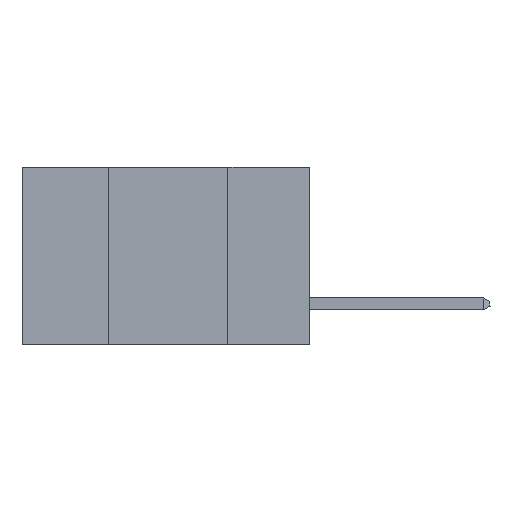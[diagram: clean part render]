
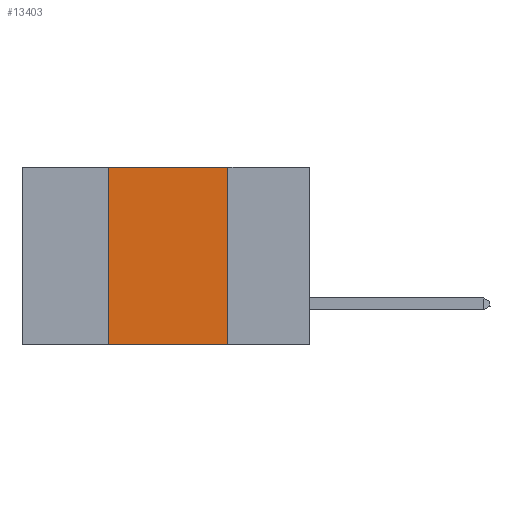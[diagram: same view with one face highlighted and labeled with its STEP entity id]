
A CAD part, left-side view. The second image highlights one B-rep face of the part: STEP entity #13403.
In plain terms, the highlighted planar face has unit normal (-1, 0, 0).
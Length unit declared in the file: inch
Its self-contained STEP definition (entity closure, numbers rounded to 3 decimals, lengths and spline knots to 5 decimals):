
#930 = EDGE_CURVE ( 'NONE', #6427, #4068, #12873, .T. ) ;
#1268 = PLANE ( 'NONE',  #1654 ) ;
#1447 = DIRECTION ( 'NONE',  ( 0., 0., 1. ) ) ;
#1532 = CARTESIAN_POINT ( 'NONE',  ( 0., 0.42, 0. ) ) ;
#1654 = AXIS2_PLACEMENT_3D ( 'NONE', #4672, #16236, #6353 ) ;
#1866 = VECTOR ( 'NONE', #7401, 39.37008 ) ;
#2319 = CARTESIAN_POINT ( 'NONE',  ( 0., 0.6, 0. ) ) ;
#2408 = VERTEX_POINT ( 'NONE', #3628 ) ;
#2888 = VECTOR ( 'NONE', #15677, 39.37008 ) ;
#2890 = EDGE_LOOP ( 'NONE', ( #3786, #19880, #3697, #14132 ) ) ;
#3628 = CARTESIAN_POINT ( 'NONE',  ( 0., 0.17, 0. ) ) ;
#3697 = ORIENTED_EDGE ( 'NONE', *, *, #21683, .F. ) ;
#3786 = ORIENTED_EDGE ( 'NONE', *, *, #4259, .F. ) ;
#4068 = VERTEX_POINT ( 'NONE', #16069 ) ;
#4259 = EDGE_CURVE ( 'NONE', #2408, #4068, #14738, .T. ) ;
#4672 = CARTESIAN_POINT ( 'NONE',  ( 0., 0.6, 0. ) ) ;
#6353 = DIRECTION ( 'NONE',  ( 0., 0., -1. ) ) ;
#6427 = VERTEX_POINT ( 'NONE', #7629 ) ;
#7181 = VERTEX_POINT ( 'NONE', #1532 ) ;
#7401 = DIRECTION ( 'NONE',  ( 0., -1., 0. ) ) ;
#7629 = CARTESIAN_POINT ( 'NONE',  ( 0., 0.42, -0.37 ) ) ;
#8702 = EDGE_CURVE ( 'NONE', #7181, #2408, #15313, .T. ) ;
#9189 = CARTESIAN_POINT ( 'NONE',  ( 0., 0.6, -0.37 ) ) ;
#11524 = CARTESIAN_POINT ( 'NONE',  ( 0., 0.42, 0. ) ) ;
#11765 = VECTOR ( 'NONE', #1447, 39.37008 ) ;
#12873 = LINE ( 'NONE', #9189, #2888 ) ;
#13403 = ADVANCED_FACE ( 'NONE', ( #17913 ), #1268, .F. ) ;
#14132 = ORIENTED_EDGE ( 'NONE', *, *, #930, .T. ) ;
#14738 = LINE ( 'NONE', #19684, #18665 ) ;
#15313 = LINE ( 'NONE', #2319, #1866 ) ;
#15677 = DIRECTION ( 'NONE',  ( 0., -1., 0. ) ) ;
#16069 = CARTESIAN_POINT ( 'NONE',  ( 0., 0.17, -0.37 ) ) ;
#16236 = DIRECTION ( 'NONE',  ( 1., 0., 0. ) ) ;
#17913 = FACE_OUTER_BOUND ( 'NONE', #2890, .T. ) ;
#18665 = VECTOR ( 'NONE', #21430, 39.37008 ) ;
#19684 = CARTESIAN_POINT ( 'NONE',  ( 0., 0.17, 0. ) ) ;
#19880 = ORIENTED_EDGE ( 'NONE', *, *, #8702, .F. ) ;
#21336 = LINE ( 'NONE', #11524, #11765 ) ;
#21430 = DIRECTION ( 'NONE',  ( 0., 0., -1. ) ) ;
#21683 = EDGE_CURVE ( 'NONE', #6427, #7181, #21336, .T. ) ;
